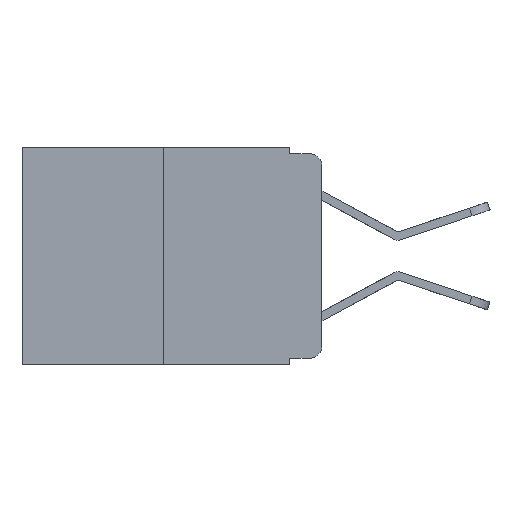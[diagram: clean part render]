
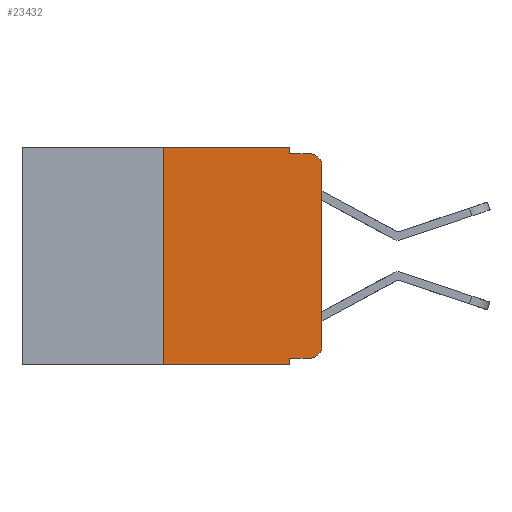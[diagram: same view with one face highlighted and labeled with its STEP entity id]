
A CAD part, left-side view. The second image highlights one B-rep face of the part: STEP entity #23432.
In plain terms, the highlighted planar face has unit normal (-1, 0, 0).
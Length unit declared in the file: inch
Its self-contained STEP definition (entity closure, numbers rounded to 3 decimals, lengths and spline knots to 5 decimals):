
#308 = LINE ( 'NONE', #24281, #13849 ) ;
#346 = CARTESIAN_POINT ( 'NONE',  ( 0., 0.051, -0.333 ) ) ;
#698 = EDGE_CURVE ( 'NONE', #14256, #19022, #19478, .T. ) ;
#918 = DIRECTION ( 'NONE',  ( -1., 0., 0. ) ) ;
#1245 = AXIS2_PLACEMENT_3D ( 'NONE', #20097, #13872, #10198 ) ;
#1734 = FACE_OUTER_BOUND ( 'NONE', #21975, .T. ) ;
#2319 = LINE ( 'NONE', #346, #5051 ) ;
#2333 = VERTEX_POINT ( 'NONE', #4435 ) ;
#2733 = CARTESIAN_POINT ( 'NONE',  ( 0., 0., 0. ) ) ;
#3473 = CARTESIAN_POINT ( 'NONE',  ( 0., 0.051, -0.01 ) ) ;
#4435 = CARTESIAN_POINT ( 'NONE',  ( 0., 0.25, -0.343 ) ) ;
#4729 = CARTESIAN_POINT ( 'NONE',  ( 0., 0.02, -0.03 ) ) ;
#4784 = VERTEX_POINT ( 'NONE', #23833 ) ;
#4916 = CARTESIAN_POINT ( 'NONE',  ( 0., 0.473, 0. ) ) ;
#5051 = VECTOR ( 'NONE', #10065, 39.37008 ) ;
#5860 = ORIENTED_EDGE ( 'NONE', *, *, #10850, .F. ) ;
#6026 = CARTESIAN_POINT ( 'NONE',  ( 0., 0.051, -0.01 ) ) ;
#6213 = DIRECTION ( 'NONE',  ( 0., 0., -1. ) ) ;
#6281 = VERTEX_POINT ( 'NONE', #11188 ) ;
#6671 = DIRECTION ( 'NONE',  ( 0., 0., 1. ) ) ;
#6905 = ORIENTED_EDGE ( 'NONE', *, *, #18134, .T. ) ;
#7098 = DIRECTION ( 'NONE',  ( 0., 0., -1. ) ) ;
#7261 = DIRECTION ( 'NONE',  ( 0., -1., 0. ) ) ;
#7295 = DIRECTION ( 'NONE',  ( 0., 0., 1. ) ) ;
#7345 = ORIENTED_EDGE ( 'NONE', *, *, #9940, .F. ) ;
#7784 = EDGE_CURVE ( 'NONE', #17880, #4784, #9221, .T. ) ;
#8010 = ORIENTED_EDGE ( 'NONE', *, *, #17871, .T. ) ;
#8491 = ORIENTED_EDGE ( 'NONE', *, *, #7784, .F. ) ;
#8652 = VECTOR ( 'NONE', #6671, 39.37008 ) ;
#9221 = LINE ( 'NONE', #4916, #11632 ) ;
#9485 = ORIENTED_EDGE ( 'NONE', *, *, #23026, .F. ) ;
#9509 = CARTESIAN_POINT ( 'NONE',  ( 0., 0.25, 0. ) ) ;
#9940 = EDGE_CURVE ( 'NONE', #20412, #6281, #25186, .T. ) ;
#10065 = DIRECTION ( 'NONE',  ( 0., -1., 0. ) ) ;
#10198 = DIRECTION ( 'NONE',  ( 0., 0., -1. ) ) ;
#10737 = PLANE ( 'NONE',  #20117 ) ;
#10850 = EDGE_CURVE ( 'NONE', #2333, #17880, #25636, .T. ) ;
#10885 = CIRCLE ( 'NONE', #25249, 0.02 ) ;
#11188 = CARTESIAN_POINT ( 'NONE',  ( 0., 0.051, -0.343 ) ) ;
#11632 = VECTOR ( 'NONE', #7261, 39.37008 ) ;
#12232 = CARTESIAN_POINT ( 'NONE',  ( 0., 0., -0.03 ) ) ;
#12256 = LINE ( 'NONE', #26022, #16305 ) ;
#12335 = CARTESIAN_POINT ( 'NONE',  ( 0., 0., -0.313 ) ) ;
#12448 = CARTESIAN_POINT ( 'NONE',  ( 0., 0.473, 0. ) ) ;
#13025 = EDGE_CURVE ( 'NONE', #19022, #17220, #14677, .T. ) ;
#13107 = DIRECTION ( 'NONE',  ( 0., 0., -1. ) ) ;
#13849 = VECTOR ( 'NONE', #22181, 39.37008 ) ;
#13872 = DIRECTION ( 'NONE',  ( -1., 0., 0. ) ) ;
#14029 = DIRECTION ( 'NONE',  ( 0., -1., 0. ) ) ;
#14256 = VERTEX_POINT ( 'NONE', #25850 ) ;
#14677 = LINE ( 'NONE', #2733, #8652 ) ;
#15236 = CARTESIAN_POINT ( 'NONE',  ( 0., 0.051, 0. ) ) ;
#15791 = CARTESIAN_POINT ( 'NONE',  ( 0., 0.051, -0.333 ) ) ;
#16265 = DIRECTION ( 'NONE',  ( 1., 0., 0. ) ) ;
#16305 = VECTOR ( 'NONE', #6213, 39.37008 ) ;
#16784 = VECTOR ( 'NONE', #14029, 39.37008 ) ;
#17220 = VERTEX_POINT ( 'NONE', #12232 ) ;
#17814 = EDGE_CURVE ( 'NONE', #20254, #21803, #24092, .T. ) ;
#17871 = EDGE_CURVE ( 'NONE', #17220, #21803, #10885, .T. ) ;
#17880 = VERTEX_POINT ( 'NONE', #22773 ) ;
#18134 = EDGE_CURVE ( 'NONE', #20412, #14256, #2319, .T. ) ;
#18391 = DIRECTION ( 'NONE',  ( 0., 0., -1. ) ) ;
#18418 = CARTESIAN_POINT ( 'NONE',  ( 0., 0.02, -0.01 ) ) ;
#18632 = EDGE_CURVE ( 'NONE', #2333, #6281, #308, .T. ) ;
#19022 = VERTEX_POINT ( 'NONE', #12335 ) ;
#19097 = ORIENTED_EDGE ( 'NONE', *, *, #13025, .T. ) ;
#19478 = CIRCLE ( 'NONE', #1245, 0.02 ) ;
#20097 = CARTESIAN_POINT ( 'NONE',  ( 0., 0.02, -0.313 ) ) ;
#20117 = AXIS2_PLACEMENT_3D ( 'NONE', #12448, #16265, #18391 ) ;
#20254 = VERTEX_POINT ( 'NONE', #3473 ) ;
#20316 = ORIENTED_EDGE ( 'NONE', *, *, #18632, .T. ) ;
#20323 = VECTOR ( 'NONE', #7098, 39.37008 ) ;
#20412 = VERTEX_POINT ( 'NONE', #15791 ) ;
#21803 = VERTEX_POINT ( 'NONE', #18418 ) ;
#21975 = EDGE_LOOP ( 'NONE', ( #19097, #8010, #23173, #9485, #8491, #5860, #20316, #7345, #6905, #23254 ) ) ;
#22046 = VECTOR ( 'NONE', #7295, 39.37008 ) ;
#22181 = DIRECTION ( 'NONE',  ( 0., -1., 0. ) ) ;
#22773 = CARTESIAN_POINT ( 'NONE',  ( 0., 0.25, 0. ) ) ;
#23026 = EDGE_CURVE ( 'NONE', #4784, #20254, #12256, .T. ) ;
#23173 = ORIENTED_EDGE ( 'NONE', *, *, #17814, .F. ) ;
#23254 = ORIENTED_EDGE ( 'NONE', *, *, #698, .T. ) ;
#23432 = ADVANCED_FACE ( 'NONE', ( #1734 ), #10737, .F. ) ;
#23833 = CARTESIAN_POINT ( 'NONE',  ( 0., 0.051, 0. ) ) ;
#24092 = LINE ( 'NONE', #6026, #16784 ) ;
#24281 = CARTESIAN_POINT ( 'NONE',  ( 0., 0.473, -0.343 ) ) ;
#25186 = LINE ( 'NONE', #15236, #20323 ) ;
#25249 = AXIS2_PLACEMENT_3D ( 'NONE', #4729, #918, #13107 ) ;
#25636 = LINE ( 'NONE', #9509, #22046 ) ;
#25850 = CARTESIAN_POINT ( 'NONE',  ( 0., 0.02, -0.333 ) ) ;
#26022 = CARTESIAN_POINT ( 'NONE',  ( 0., 0.051, 0. ) ) ;
